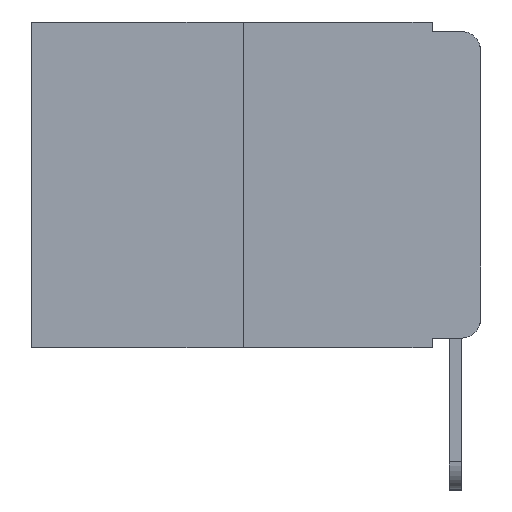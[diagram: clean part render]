
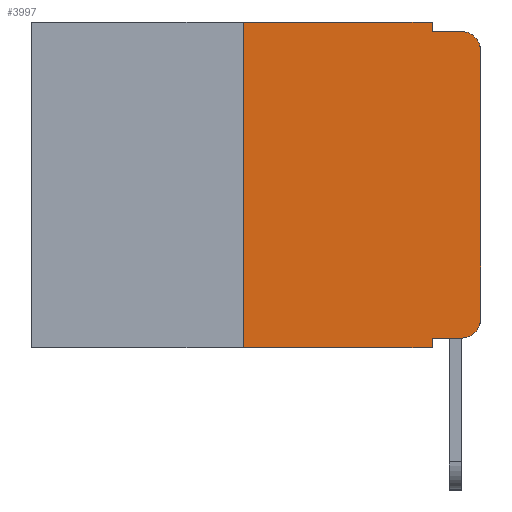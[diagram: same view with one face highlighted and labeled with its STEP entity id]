
A CAD part, left-side view. The second image highlights one B-rep face of the part: STEP entity #3997.
In plain terms, the highlighted planar face has unit normal (-1, 0, 0).
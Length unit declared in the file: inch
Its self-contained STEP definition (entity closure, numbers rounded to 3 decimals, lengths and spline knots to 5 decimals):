
#23 = ORIENTED_EDGE ( 'NONE', *, *, #7013, .F. ) ;
#192 = DIRECTION ( 'NONE',  ( 0., 0., -1. ) ) ;
#422 = CARTESIAN_POINT ( 'NONE',  ( 0., 0.25, 0. ) ) ;
#459 = CIRCLE ( 'NONE', #11906, 0.02 ) ;
#487 = EDGE_CURVE ( 'NONE', #4981, #10372, #9483, .T. ) ;
#534 = VERTEX_POINT ( 'NONE', #4366 ) ;
#588 = EDGE_LOOP ( 'NONE', ( #1948, #13301, #13598, #9044, #4419, #7921, #7933, #23, #9217, #1565 ) ) ;
#703 = VECTOR ( 'NONE', #4474, 39.37008 ) ;
#837 = VERTEX_POINT ( 'NONE', #3854 ) ;
#1190 = DIRECTION ( 'NONE',  ( 0., 0., -1. ) ) ;
#1211 = DIRECTION ( 'NONE',  ( 1., 0., 0. ) ) ;
#1215 = PLANE ( 'NONE',  #5206 ) ;
#1413 = VERTEX_POINT ( 'NONE', #9205 ) ;
#1484 = VECTOR ( 'NONE', #4903, 39.37008 ) ;
#1565 = ORIENTED_EDGE ( 'NONE', *, *, #7671, .T. ) ;
#1755 = EDGE_CURVE ( 'NONE', #10372, #4423, #10855, .T. ) ;
#1879 = CARTESIAN_POINT ( 'NONE',  ( 0., 0.473, 0. ) ) ;
#1918 = CARTESIAN_POINT ( 'NONE',  ( 0., 0.02, -0.313 ) ) ;
#1948 = ORIENTED_EDGE ( 'NONE', *, *, #13157, .T. ) ;
#2471 = VERTEX_POINT ( 'NONE', #10696 ) ;
#2582 = VECTOR ( 'NONE', #13519, 39.37008 ) ;
#2638 = VECTOR ( 'NONE', #9237, 39.37008 ) ;
#3067 = DIRECTION ( 'NONE',  ( 0., 0., -1. ) ) ;
#3328 = CARTESIAN_POINT ( 'NONE',  ( 0., 0.051, 0. ) ) ;
#3337 = CARTESIAN_POINT ( 'NONE',  ( 0., 0.051, -0.333 ) ) ;
#3346 = DIRECTION ( 'NONE',  ( 0., 0., -1. ) ) ;
#3497 = CARTESIAN_POINT ( 'NONE',  ( 0., 0.02, -0.01 ) ) ;
#3629 = CARTESIAN_POINT ( 'NONE',  ( 0., 0.25, 0. ) ) ;
#3793 = CARTESIAN_POINT ( 'NONE',  ( 0., 0.473, -0.343 ) ) ;
#3854 = CARTESIAN_POINT ( 'NONE',  ( 0., 0.02, -0.333 ) ) ;
#3997 = ADVANCED_FACE ( 'NONE', ( #7763 ), #1215, .F. ) ;
#4366 = CARTESIAN_POINT ( 'NONE',  ( 0., 0.051, -0.343 ) ) ;
#4419 = ORIENTED_EDGE ( 'NONE', *, *, #487, .F. ) ;
#4423 = VERTEX_POINT ( 'NONE', #7965 ) ;
#4474 = DIRECTION ( 'NONE',  ( 0., -1., 0. ) ) ;
#4895 = VERTEX_POINT ( 'NONE', #3497 ) ;
#4903 = DIRECTION ( 'NONE',  ( 0., -1., 0. ) ) ;
#4981 = VERTEX_POINT ( 'NONE', #3629 ) ;
#5206 = AXIS2_PLACEMENT_3D ( 'NONE', #7372, #1211, #1190 ) ;
#5280 = AXIS2_PLACEMENT_3D ( 'NONE', #12958, #6955, #192 ) ;
#5424 = CARTESIAN_POINT ( 'NONE',  ( 0., 0.051, 0. ) ) ;
#5553 = VECTOR ( 'NONE', #7500, 39.37008 ) ;
#5574 = VERTEX_POINT ( 'NONE', #10938 ) ;
#5875 = LINE ( 'NONE', #5424, #5553 ) ;
#5909 = LINE ( 'NONE', #11179, #2638 ) ;
#6551 = LINE ( 'NONE', #9866, #9004 ) ;
#6771 = EDGE_CURVE ( 'NONE', #2471, #4981, #8503, .T. ) ;
#6955 = DIRECTION ( 'NONE',  ( -1., 0., 0. ) ) ;
#7013 = EDGE_CURVE ( 'NONE', #1413, #534, #5875, .T. ) ;
#7350 = EDGE_CURVE ( 'NONE', #1413, #837, #10993, .T. ) ;
#7372 = CARTESIAN_POINT ( 'NONE',  ( 0., 0.473, 0. ) ) ;
#7500 = DIRECTION ( 'NONE',  ( 0., 0., -1. ) ) ;
#7618 = CARTESIAN_POINT ( 'NONE',  ( 0., 0.051, 0. ) ) ;
#7671 = EDGE_CURVE ( 'NONE', #837, #5574, #459, .T. ) ;
#7763 = FACE_OUTER_BOUND ( 'NONE', #588, .T. ) ;
#7921 = ORIENTED_EDGE ( 'NONE', *, *, #6771, .F. ) ;
#7933 = ORIENTED_EDGE ( 'NONE', *, *, #13387, .T. ) ;
#7965 = CARTESIAN_POINT ( 'NONE',  ( 0., 0.051, -0.01 ) ) ;
#8503 = LINE ( 'NONE', #422, #13396 ) ;
#9004 = VECTOR ( 'NONE', #9822, 39.37008 ) ;
#9044 = ORIENTED_EDGE ( 'NONE', *, *, #1755, .F. ) ;
#9205 = CARTESIAN_POINT ( 'NONE',  ( 0., 0.051, -0.333 ) ) ;
#9217 = ORIENTED_EDGE ( 'NONE', *, *, #7350, .T. ) ;
#9237 = DIRECTION ( 'NONE',  ( 0., -1., 0. ) ) ;
#9453 = DIRECTION ( 'NONE',  ( -1., 0., 0. ) ) ;
#9483 = LINE ( 'NONE', #1879, #703 ) ;
#9822 = DIRECTION ( 'NONE',  ( 0., 0., 1. ) ) ;
#9866 = CARTESIAN_POINT ( 'NONE',  ( 0., 0., 0. ) ) ;
#10104 = LINE ( 'NONE', #3793, #1484 ) ;
#10263 = DIRECTION ( 'NONE',  ( 0., 0., 1. ) ) ;
#10372 = VERTEX_POINT ( 'NONE', #7618 ) ;
#10592 = CIRCLE ( 'NONE', #5280, 0.02 ) ;
#10696 = CARTESIAN_POINT ( 'NONE',  ( 0., 0.25, -0.343 ) ) ;
#10855 = LINE ( 'NONE', #3328, #13105 ) ;
#10938 = CARTESIAN_POINT ( 'NONE',  ( 0., 0., -0.313 ) ) ;
#10993 = LINE ( 'NONE', #3337, #2582 ) ;
#11179 = CARTESIAN_POINT ( 'NONE',  ( 0., 0.051, -0.01 ) ) ;
#11502 = CARTESIAN_POINT ( 'NONE',  ( 0., 0., -0.03 ) ) ;
#11648 = VERTEX_POINT ( 'NONE', #11502 ) ;
#11906 = AXIS2_PLACEMENT_3D ( 'NONE', #1918, #9453, #3067 ) ;
#12550 = EDGE_CURVE ( 'NONE', #11648, #4895, #10592, .T. ) ;
#12713 = EDGE_CURVE ( 'NONE', #4423, #4895, #5909, .T. ) ;
#12958 = CARTESIAN_POINT ( 'NONE',  ( 0., 0.02, -0.03 ) ) ;
#13105 = VECTOR ( 'NONE', #3346, 39.37008 ) ;
#13157 = EDGE_CURVE ( 'NONE', #5574, #11648, #6551, .T. ) ;
#13301 = ORIENTED_EDGE ( 'NONE', *, *, #12550, .T. ) ;
#13387 = EDGE_CURVE ( 'NONE', #2471, #534, #10104, .T. ) ;
#13396 = VECTOR ( 'NONE', #10263, 39.37008 ) ;
#13519 = DIRECTION ( 'NONE',  ( 0., -1., 0. ) ) ;
#13598 = ORIENTED_EDGE ( 'NONE', *, *, #12713, .F. ) ;
